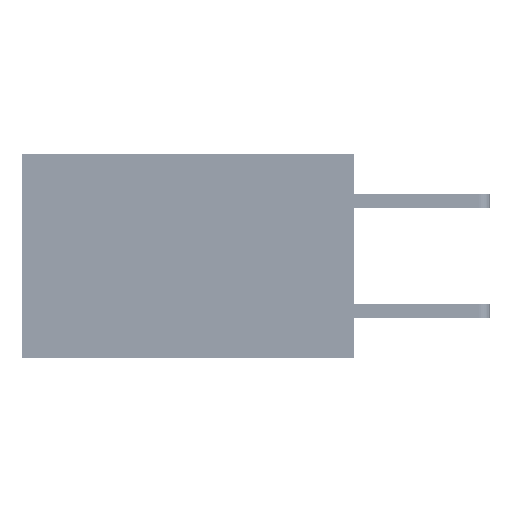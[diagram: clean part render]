
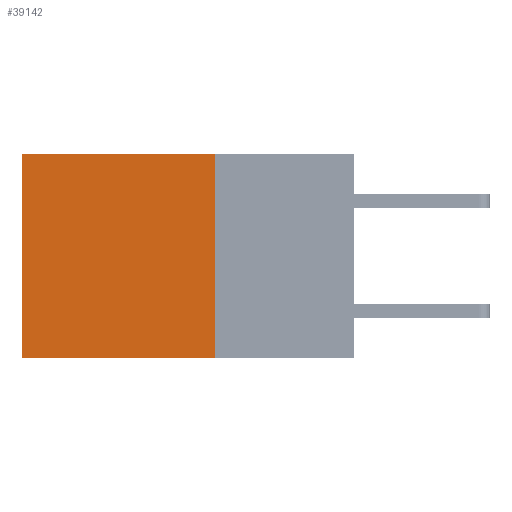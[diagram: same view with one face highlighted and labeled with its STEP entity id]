
A CAD part, left-side view. The second image highlights one B-rep face of the part: STEP entity #39142.
In plain terms, the highlighted planar face has unit normal (-1, 0, 0).
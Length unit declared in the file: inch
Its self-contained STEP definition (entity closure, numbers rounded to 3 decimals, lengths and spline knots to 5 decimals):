
#1242 = LINE ( 'NONE', #8253, #19197 ) ;
#2023 = DIRECTION ( 'NONE',  ( 0., 0., -1. ) ) ;
#3134 = ORIENTED_EDGE ( 'NONE', *, *, #8903, .T. ) ;
#5486 = VERTEX_POINT ( 'NONE', #22335 ) ;
#5530 = CARTESIAN_POINT ( 'NONE',  ( 0.2875, 0.25, 0. ) ) ;
#6409 = CARTESIAN_POINT ( 'NONE',  ( 0.2875, 0.25, -0.37 ) ) ;
#8253 = CARTESIAN_POINT ( 'NONE',  ( 0.2875, 0.25, 0. ) ) ;
#8602 = FACE_OUTER_BOUND ( 'NONE', #20206, .T. ) ;
#8903 = EDGE_CURVE ( 'NONE', #27580, #10544, #1242, .T. ) ;
#10544 = VERTEX_POINT ( 'NONE', #36114 ) ;
#12325 = VERTEX_POINT ( 'NONE', #34517 ) ;
#13961 = EDGE_CURVE ( 'NONE', #12325, #5486, #39747, .T. ) ;
#16474 = VECTOR ( 'NONE', #22705, 39.37008 ) ;
#16516 = DIRECTION ( 'NONE',  ( 0., 1., 0. ) ) ;
#18583 = EDGE_CURVE ( 'NONE', #10544, #5486, #38093, .T. ) ;
#19197 = VECTOR ( 'NONE', #28444, 39.37008 ) ;
#20206 = EDGE_LOOP ( 'NONE', ( #42799, #21553, #24862, #3134 ) ) ;
#20753 = EDGE_CURVE ( 'NONE', #27580, #12325, #25994, .T. ) ;
#21553 = ORIENTED_EDGE ( 'NONE', *, *, #13961, .F. ) ;
#22335 = CARTESIAN_POINT ( 'NONE',  ( 0.2875, 0.6, -0.37 ) ) ;
#22705 = DIRECTION ( 'NONE',  ( 0., 0., -1. ) ) ;
#24862 = ORIENTED_EDGE ( 'NONE', *, *, #20753, .F. ) ;
#25501 = PLANE ( 'NONE',  #38809 ) ;
#25794 = CARTESIAN_POINT ( 'NONE',  ( 0.2875, 0.25, 0. ) ) ;
#25994 = LINE ( 'NONE', #25794, #16474 ) ;
#27580 = VERTEX_POINT ( 'NONE', #43127 ) ;
#27801 = DIRECTION ( 'NONE',  ( 0., 0., -1. ) ) ;
#28444 = DIRECTION ( 'NONE',  ( 0., 1., 0. ) ) ;
#29534 = VECTOR ( 'NONE', #27801, 39.37008 ) ;
#31712 = CARTESIAN_POINT ( 'NONE',  ( 0.2875, 0.6, 0. ) ) ;
#34517 = CARTESIAN_POINT ( 'NONE',  ( 0.2875, 0.25, -0.37 ) ) ;
#36114 = CARTESIAN_POINT ( 'NONE',  ( 0.2875, 0.6, 0. ) ) ;
#36641 = VECTOR ( 'NONE', #16516, 39.37008 ) ;
#38093 = LINE ( 'NONE', #31712, #29534 ) ;
#38809 = AXIS2_PLACEMENT_3D ( 'NONE', #5530, #39078, #2023 ) ;
#39078 = DIRECTION ( 'NONE',  ( 1., 0., 0. ) ) ;
#39142 = ADVANCED_FACE ( 'NONE', ( #8602 ), #25501, .F. ) ;
#39747 = LINE ( 'NONE', #6409, #36641 ) ;
#42799 = ORIENTED_EDGE ( 'NONE', *, *, #18583, .T. ) ;
#43127 = CARTESIAN_POINT ( 'NONE',  ( 0.2875, 0.25, 0. ) ) ;
